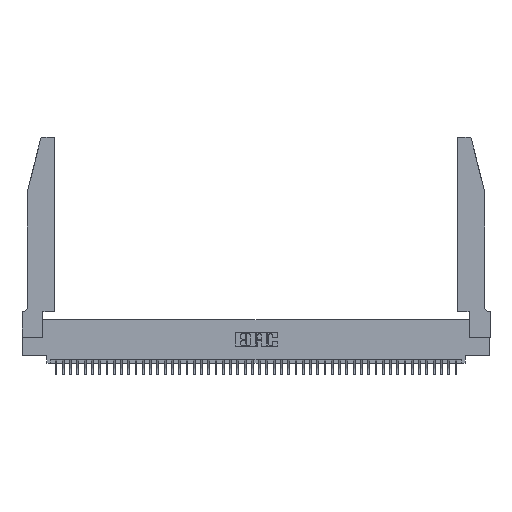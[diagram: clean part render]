
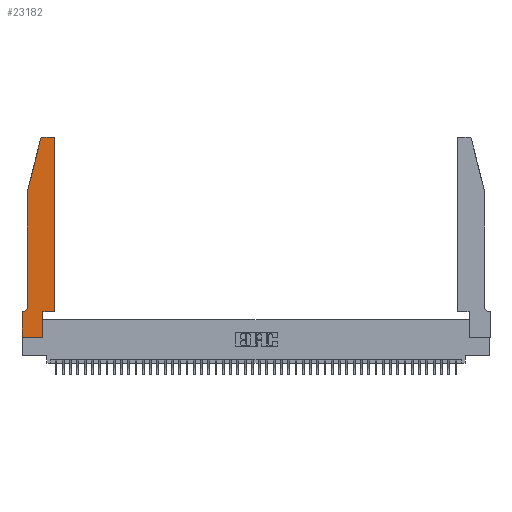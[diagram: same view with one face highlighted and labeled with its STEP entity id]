
A CAD part, top view. The second image highlights one B-rep face of the part: STEP entity #23182.
In plain terms, the highlighted planar face has unit normal (0, 0, 1).
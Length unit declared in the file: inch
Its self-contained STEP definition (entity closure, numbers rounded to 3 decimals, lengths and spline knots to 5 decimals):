
#25 = CARTESIAN_POINT ( 'NONE',  ( 0.284, 2.72, 0.37 ) ) ;
#128 = DIRECTION ( 'NONE',  ( -1., 0., 0. ) ) ;
#234 = FACE_OUTER_BOUND ( 'NONE', #42144, .T. ) ;
#374 = VECTOR ( 'NONE', #36078, 39.37008 ) ;
#1352 = LINE ( 'NONE', #25763, #45258 ) ;
#1703 = VERTEX_POINT ( 'NONE', #44219 ) ;
#2616 = ORIENTED_EDGE ( 'NONE', *, *, #31731, .T. ) ;
#2883 = ORIENTED_EDGE ( 'NONE', *, *, #46905, .T. ) ;
#4546 = VERTEX_POINT ( 'NONE', #6558 ) ;
#5062 = VERTEX_POINT ( 'NONE', #8552 ) ;
#5188 = CARTESIAN_POINT ( 'NONE',  ( 0.4505, 0.35, 0.37 ) ) ;
#5367 = EDGE_CURVE ( 'NONE', #24487, #40623, #17625, .T. ) ;
#5962 = ORIENTED_EDGE ( 'NONE', *, *, #27848, .T. ) ;
#6495 = LINE ( 'NONE', #45882, #22465 ) ;
#6496 = DIRECTION ( 'NONE',  ( -0.239, -0.971, 0. ) ) ;
#6558 = CARTESIAN_POINT ( 'NONE',  ( 0.2865, 0.35, 0.37 ) ) ;
#6932 = ORIENTED_EDGE ( 'NONE', *, *, #11269, .T. ) ;
#7198 = CARTESIAN_POINT ( 'NONE',  ( 0.4505, 0.35, 0.37 ) ) ;
#8552 = CARTESIAN_POINT ( 'NONE',  ( 0.0755, 2., 0.37 ) ) ;
#9254 = AXIS2_PLACEMENT_3D ( 'NONE', #34885, #31544, #42538 ) ;
#9922 = CARTESIAN_POINT ( 'NONE',  ( 0.4205, 2.72, 0.37 ) ) ;
#10654 = CARTESIAN_POINT ( 'NONE',  ( 0.4205, 2.75, 0.37 ) ) ;
#11217 = VECTOR ( 'NONE', #17123, 39.37008 ) ;
#11269 = EDGE_CURVE ( 'NONE', #5062, #24487, #35225, .T. ) ;
#12793 = CIRCLE ( 'NONE', #46370, 0.03 ) ;
#14095 = VERTEX_POINT ( 'NONE', #29610 ) ;
#14435 = ORIENTED_EDGE ( 'NONE', *, *, #39972, .T. ) ;
#15500 = ORIENTED_EDGE ( 'NONE', *, *, #39150, .T. ) ;
#16237 = ORIENTED_EDGE ( 'NONE', *, *, #5367, .T. ) ;
#16364 = CARTESIAN_POINT ( 'NONE',  ( 0., 0.35, 0.37 ) ) ;
#16588 = VECTOR ( 'NONE', #128, 39.37008 ) ;
#16659 = CARTESIAN_POINT ( 'NONE',  ( 0.2865, 0., 0.37 ) ) ;
#16809 = AXIS2_PLACEMENT_3D ( 'NONE', #9922, #20914, #39195 ) ;
#17123 = DIRECTION ( 'NONE',  ( 1., 0., 0. ) ) ;
#17625 = CIRCLE ( 'NONE', #9254, 0.07 ) ;
#17813 = ORIENTED_EDGE ( 'NONE', *, *, #42256, .T. ) ;
#18065 = AXIS2_PLACEMENT_3D ( 'NONE', #16364, #41826, #45631 ) ;
#18460 = VECTOR ( 'NONE', #39498, 39.37008 ) ;
#18919 = ORIENTED_EDGE ( 'NONE', *, *, #40999, .T. ) ;
#20914 = DIRECTION ( 'NONE',  ( 0., 0., 1. ) ) ;
#21146 = VERTEX_POINT ( 'NONE', #7198 ) ;
#21784 = CARTESIAN_POINT ( 'NONE',  ( 0.0755, 2., 0.37 ) ) ;
#22465 = VECTOR ( 'NONE', #23769, 39.37008 ) ;
#23182 = ADVANCED_FACE ( 'NONE', ( #234 ), #34445, .T. ) ;
#23695 = EDGE_CURVE ( 'NONE', #38849, #5062, #36458, .T. ) ;
#23769 = DIRECTION ( 'NONE',  ( 0., 1., 0. ) ) ;
#24487 = VERTEX_POINT ( 'NONE', #40495 ) ;
#24490 = CARTESIAN_POINT ( 'NONE',  ( 0.0055, 0.35, 0.37 ) ) ;
#25763 = CARTESIAN_POINT ( 'NONE',  ( 0., 0., 0.37 ) ) ;
#25906 = DIRECTION ( 'NONE',  ( 1., 0., 0. ) ) ;
#27764 = VECTOR ( 'NONE', #30961, 39.37008 ) ;
#27848 = EDGE_CURVE ( 'NONE', #41198, #4546, #43219, .T. ) ;
#29064 = VERTEX_POINT ( 'NONE', #40336 ) ;
#29275 = DIRECTION ( 'NONE',  ( 1., 0., 0. ) ) ;
#29610 = CARTESIAN_POINT ( 'NONE',  ( 0., 0., 0.37 ) ) ;
#30961 = DIRECTION ( 'NONE',  ( 0., -1., 0. ) ) ;
#31233 = ORIENTED_EDGE ( 'NONE', *, *, #23695, .T. ) ;
#31544 = DIRECTION ( 'NONE',  ( 0., 0., -1. ) ) ;
#31703 = VERTEX_POINT ( 'NONE', #38402 ) ;
#31731 = EDGE_CURVE ( 'NONE', #21146, #29064, #6495, .T. ) ;
#31863 = CIRCLE ( 'NONE', #16809, 0.03 ) ;
#32483 = ORIENTED_EDGE ( 'NONE', *, *, #36339, .T. ) ;
#33508 = VECTOR ( 'NONE', #6496, 39.37008 ) ;
#34278 = CARTESIAN_POINT ( 'NONE',  ( 0.0755, 0.35, 0.37 ) ) ;
#34445 = PLANE ( 'NONE',  #18065 ) ;
#34885 = CARTESIAN_POINT ( 'NONE',  ( 0.0055, 0.42, 0.37 ) ) ;
#35225 = LINE ( 'NONE', #21784, #374 ) ;
#35678 = CARTESIAN_POINT ( 'NONE',  ( 0.2605, 2.75, 0.37 ) ) ;
#35693 = LINE ( 'NONE', #5188, #11217 ) ;
#36078 = DIRECTION ( 'NONE',  ( 0., -1., 0. ) ) ;
#36339 = EDGE_CURVE ( 'NONE', #4546, #21146, #35693, .T. ) ;
#36458 = LINE ( 'NONE', #43209, #33508 ) ;
#36553 = ORIENTED_EDGE ( 'NONE', *, *, #42566, .T. ) ;
#38060 = LINE ( 'NONE', #44020, #27764 ) ;
#38402 = CARTESIAN_POINT ( 'NONE',  ( 0., 0.35, 0.37 ) ) ;
#38849 = VERTEX_POINT ( 'NONE', #41433 ) ;
#38970 = LINE ( 'NONE', #35678, #18460 ) ;
#39150 = EDGE_CURVE ( 'NONE', #40623, #31703, #40431, .T. ) ;
#39195 = DIRECTION ( 'NONE',  ( 1., 0., 0. ) ) ;
#39498 = DIRECTION ( 'NONE',  ( -1., 0., 0. ) ) ;
#39972 = EDGE_CURVE ( 'NONE', #29064, #43171, #31863, .T. ) ;
#40135 = DIRECTION ( 'NONE',  ( 0., 0., 1. ) ) ;
#40336 = CARTESIAN_POINT ( 'NONE',  ( 0.4505, 2.72, 0.37 ) ) ;
#40431 = LINE ( 'NONE', #34278, #16588 ) ;
#40495 = CARTESIAN_POINT ( 'NONE',  ( 0.0755, 0.42, 0.37 ) ) ;
#40590 = DIRECTION ( 'NONE',  ( 0., 1., 0. ) ) ;
#40623 = VERTEX_POINT ( 'NONE', #24490 ) ;
#40999 = EDGE_CURVE ( 'NONE', #31703, #14095, #38060, .T. ) ;
#41198 = VERTEX_POINT ( 'NONE', #16659 ) ;
#41433 = CARTESIAN_POINT ( 'NONE',  ( 0.25487, 2.72718, 0.37 ) ) ;
#41826 = DIRECTION ( 'NONE',  ( 0., 0., 1. ) ) ;
#42144 = EDGE_LOOP ( 'NONE', ( #36553, #2883, #31233, #6932, #16237, #15500, #18919, #17813, #5962, #32483, #2616, #14435 ) ) ;
#42256 = EDGE_CURVE ( 'NONE', #14095, #41198, #1352, .T. ) ;
#42538 = DIRECTION ( 'NONE',  ( -1., 0., 0. ) ) ;
#42566 = EDGE_CURVE ( 'NONE', #43171, #1703, #38970, .T. ) ;
#43171 = VERTEX_POINT ( 'NONE', #10654 ) ;
#43209 = CARTESIAN_POINT ( 'NONE',  ( 0.0755, 2., 0.37 ) ) ;
#43219 = LINE ( 'NONE', #44109, #46661 ) ;
#44020 = CARTESIAN_POINT ( 'NONE',  ( 0., 0., 0.37 ) ) ;
#44109 = CARTESIAN_POINT ( 'NONE',  ( 0.2865, 0.35, 0.37 ) ) ;
#44219 = CARTESIAN_POINT ( 'NONE',  ( 0.284, 2.75, 0.37 ) ) ;
#45258 = VECTOR ( 'NONE', #25906, 39.37008 ) ;
#45631 = DIRECTION ( 'NONE',  ( 1., 0., 0. ) ) ;
#45882 = CARTESIAN_POINT ( 'NONE',  ( 0.4505, 0.35, 0.37 ) ) ;
#46370 = AXIS2_PLACEMENT_3D ( 'NONE', #25, #40135, #29275 ) ;
#46661 = VECTOR ( 'NONE', #40590, 39.37008 ) ;
#46905 = EDGE_CURVE ( 'NONE', #1703, #38849, #12793, .T. ) ;
